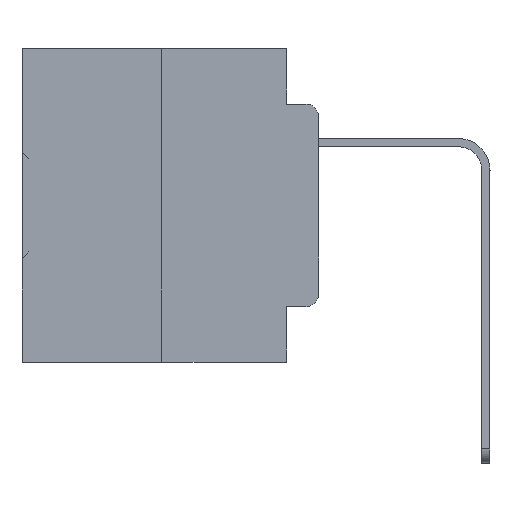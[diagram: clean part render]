
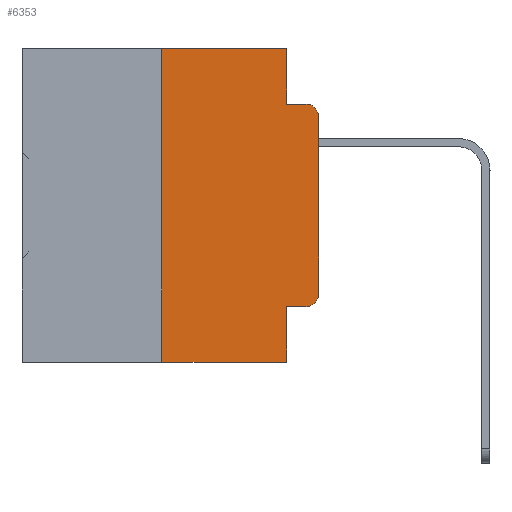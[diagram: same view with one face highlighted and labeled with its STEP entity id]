
A CAD part, left-side view. The second image highlights one B-rep face of the part: STEP entity #6353.
In plain terms, the highlighted planar face has unit normal (-1, 0, 0).
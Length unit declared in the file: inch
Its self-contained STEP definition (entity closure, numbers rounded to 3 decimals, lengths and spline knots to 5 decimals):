
#112 = ORIENTED_EDGE ( 'NONE', *, *, #838, .F. ) ;
#681 = EDGE_LOOP ( 'NONE', ( #30294, #35174, #11820, #36654, #112, #9363, #1224, #33022, #19173, #34422 ) ) ;
#756 = CIRCLE ( 'NONE', #16115, 0.02 ) ;
#838 = EDGE_CURVE ( 'NONE', #27940, #31191, #33727, .T. ) ;
#1215 = EDGE_CURVE ( 'NONE', #31191, #13922, #21193, .T. ) ;
#1224 = ORIENTED_EDGE ( 'NONE', *, *, #18741, .T. ) ;
#2147 = EDGE_CURVE ( 'NONE', #6208, #28122, #29567, .T. ) ;
#2734 = CARTESIAN_POINT ( 'NONE',  ( 0., 0., -0.3915 ) ) ;
#2956 = CARTESIAN_POINT ( 'NONE',  ( 0., 0.02, -0.4115 ) ) ;
#3294 = VERTEX_POINT ( 'NONE', #5100 ) ;
#3897 = EDGE_CURVE ( 'NONE', #28122, #13160, #18028, .T. ) ;
#4057 = CARTESIAN_POINT ( 'NONE',  ( 0., 0.02, -0.3915 ) ) ;
#5100 = CARTESIAN_POINT ( 'NONE',  ( 0., 0.051, -0.5 ) ) ;
#5640 = CARTESIAN_POINT ( 'NONE',  ( 0., 0.051, -0.4115 ) ) ;
#5896 = FACE_OUTER_BOUND ( 'NONE', #681, .T. ) ;
#6095 = CARTESIAN_POINT ( 'NONE',  ( 0., 0.051, 0. ) ) ;
#6208 = VERTEX_POINT ( 'NONE', #5640 ) ;
#6353 = ADVANCED_FACE ( 'NONE', ( #5896 ), #28865, .F. ) ;
#6658 = LINE ( 'NONE', #18671, #27571 ) ;
#6872 = DIRECTION ( 'NONE',  ( -1., 0., 0. ) ) ;
#6899 = LINE ( 'NONE', #6095, #7810 ) ;
#7043 = CARTESIAN_POINT ( 'NONE',  ( 0., 0., 0. ) ) ;
#7736 = VECTOR ( 'NONE', #19581, 39.37008 ) ;
#7793 = EDGE_CURVE ( 'NONE', #13922, #12855, #6658, .T. ) ;
#7810 = VECTOR ( 'NONE', #9322, 39.37008 ) ;
#9322 = DIRECTION ( 'NONE',  ( 0., 0., -1. ) ) ;
#9329 = DIRECTION ( 'NONE',  ( 0., 0., -1. ) ) ;
#9363 = ORIENTED_EDGE ( 'NONE', *, *, #13151, .F. ) ;
#9660 = LINE ( 'NONE', #24320, #18103 ) ;
#9742 = CARTESIAN_POINT ( 'NONE',  ( 0., 0., -0.1085 ) ) ;
#10416 = AXIS2_PLACEMENT_3D ( 'NONE', #17658, #34610, #9329 ) ;
#11444 = VECTOR ( 'NONE', #35337, 39.37008 ) ;
#11820 = ORIENTED_EDGE ( 'NONE', *, *, #7793, .F. ) ;
#12321 = CARTESIAN_POINT ( 'NONE',  ( 0., 0.02, -0.1085 ) ) ;
#12527 = DIRECTION ( 'NONE',  ( 0., 0., 1. ) ) ;
#12855 = VERTEX_POINT ( 'NONE', #23471 ) ;
#13151 = EDGE_CURVE ( 'NONE', #35999, #27940, #9660, .T. ) ;
#13160 = VERTEX_POINT ( 'NONE', #2734 ) ;
#13922 = VERTEX_POINT ( 'NONE', #32137 ) ;
#14604 = DIRECTION ( 'NONE',  ( 0., -1., 0. ) ) ;
#15294 = DIRECTION ( 'NONE',  ( 0., 0., -1. ) ) ;
#16115 = AXIS2_PLACEMENT_3D ( 'NONE', #12321, #24641, #15294 ) ;
#17298 = EDGE_CURVE ( 'NONE', #28214, #12855, #756, .T. ) ;
#17568 = VECTOR ( 'NONE', #14604, 39.37008 ) ;
#17658 = CARTESIAN_POINT ( 'NONE',  ( 0., 0.473, 0. ) ) ;
#17666 = EDGE_CURVE ( 'NONE', #6208, #3294, #6899, .T. ) ;
#17719 = CARTESIAN_POINT ( 'NONE',  ( 0., 0.051, 0. ) ) ;
#18028 = CIRCLE ( 'NONE', #36594, 0.02 ) ;
#18103 = VECTOR ( 'NONE', #27314, 39.37008 ) ;
#18671 = CARTESIAN_POINT ( 'NONE',  ( 0., 0.051, -0.0885 ) ) ;
#18741 = EDGE_CURVE ( 'NONE', #35999, #3294, #20606, .T. ) ;
#19173 = ORIENTED_EDGE ( 'NONE', *, *, #2147, .T. ) ;
#19431 = DIRECTION ( 'NONE',  ( 0., -1., 0. ) ) ;
#19581 = DIRECTION ( 'NONE',  ( 0., -1., 0. ) ) ;
#19674 = EDGE_CURVE ( 'NONE', #13160, #28214, #30807, .T. ) ;
#20606 = LINE ( 'NONE', #28152, #7736 ) ;
#21193 = LINE ( 'NONE', #26833, #11444 ) ;
#23471 = CARTESIAN_POINT ( 'NONE',  ( 0., 0.02, -0.0885 ) ) ;
#24320 = CARTESIAN_POINT ( 'NONE',  ( 0., 0.25, 0. ) ) ;
#24641 = DIRECTION ( 'NONE',  ( -1., 0., 0. ) ) ;
#25425 = CARTESIAN_POINT ( 'NONE',  ( 0., 0.25, 0. ) ) ;
#25914 = CARTESIAN_POINT ( 'NONE',  ( 0., 0.051, -0.4115 ) ) ;
#26764 = VECTOR ( 'NONE', #12527, 39.37008 ) ;
#26833 = CARTESIAN_POINT ( 'NONE',  ( 0., 0.051, 0. ) ) ;
#26978 = DIRECTION ( 'NONE',  ( 0., -1., 0. ) ) ;
#27314 = DIRECTION ( 'NONE',  ( 0., 0., 1. ) ) ;
#27571 = VECTOR ( 'NONE', #26978, 39.37008 ) ;
#27749 = CARTESIAN_POINT ( 'NONE',  ( 0., 0.473, 0. ) ) ;
#27940 = VERTEX_POINT ( 'NONE', #25425 ) ;
#28122 = VERTEX_POINT ( 'NONE', #2956 ) ;
#28152 = CARTESIAN_POINT ( 'NONE',  ( 0., 0.473, -0.5 ) ) ;
#28214 = VERTEX_POINT ( 'NONE', #9742 ) ;
#28865 = PLANE ( 'NONE',  #10416 ) ;
#29057 = CARTESIAN_POINT ( 'NONE',  ( 0., 0.25, -0.5 ) ) ;
#29567 = LINE ( 'NONE', #25914, #17568 ) ;
#29617 = DIRECTION ( 'NONE',  ( 0., 0., -1. ) ) ;
#30294 = ORIENTED_EDGE ( 'NONE', *, *, #19674, .T. ) ;
#30807 = LINE ( 'NONE', #7043, #26764 ) ;
#31191 = VERTEX_POINT ( 'NONE', #17719 ) ;
#32137 = CARTESIAN_POINT ( 'NONE',  ( 0., 0.051, -0.0885 ) ) ;
#33022 = ORIENTED_EDGE ( 'NONE', *, *, #17666, .F. ) ;
#33727 = LINE ( 'NONE', #27749, #34633 ) ;
#34422 = ORIENTED_EDGE ( 'NONE', *, *, #3897, .T. ) ;
#34610 = DIRECTION ( 'NONE',  ( 1., 0., 0. ) ) ;
#34633 = VECTOR ( 'NONE', #19431, 39.37008 ) ;
#35174 = ORIENTED_EDGE ( 'NONE', *, *, #17298, .T. ) ;
#35337 = DIRECTION ( 'NONE',  ( 0., 0., -1. ) ) ;
#35999 = VERTEX_POINT ( 'NONE', #29057 ) ;
#36594 = AXIS2_PLACEMENT_3D ( 'NONE', #4057, #6872, #29617 ) ;
#36654 = ORIENTED_EDGE ( 'NONE', *, *, #1215, .F. ) ;
